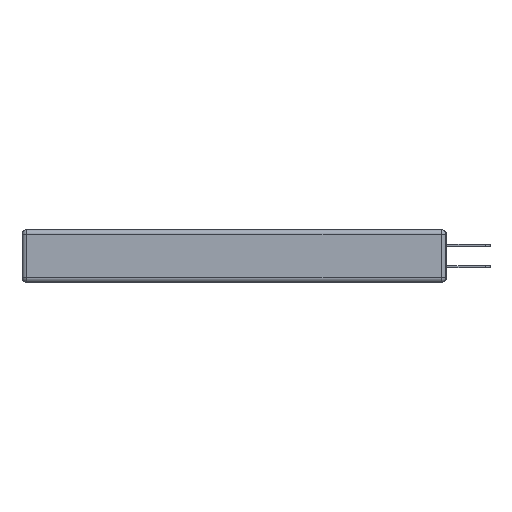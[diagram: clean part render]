
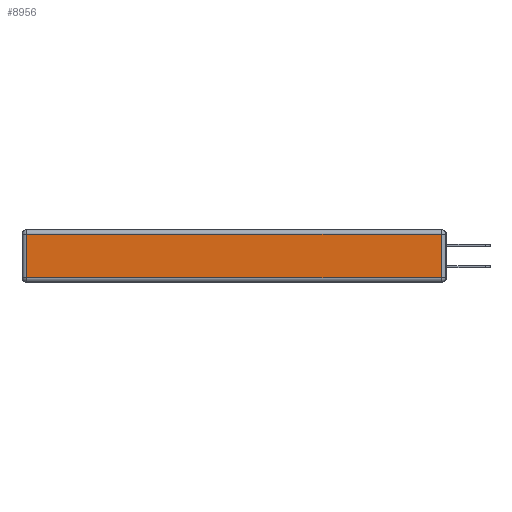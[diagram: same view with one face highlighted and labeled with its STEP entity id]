
A CAD part, left-side view. The second image highlights one B-rep face of the part: STEP entity #8956.
In plain terms, the highlighted planar face has unit normal (-1, 0, 0).
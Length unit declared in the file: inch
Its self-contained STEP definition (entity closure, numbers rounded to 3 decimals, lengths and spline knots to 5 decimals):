
#381 = CARTESIAN_POINT ( 'NONE',  ( 0., 2.72, -0.343 ) ) ;
#869 = DIRECTION ( 'NONE',  ( 0., 0., 1. ) ) ;
#1043 = LINE ( 'NONE', #381, #15610 ) ;
#2469 = DIRECTION ( 'NONE',  ( -1., 0., 0. ) ) ;
#3459 = LINE ( 'NONE', #8683, #8303 ) ;
#4375 = VECTOR ( 'NONE', #24062, 39.37008 ) ;
#4778 = CARTESIAN_POINT ( 'NONE',  ( 0., 2.72, -0.03 ) ) ;
#6944 = AXIS2_PLACEMENT_3D ( 'NONE', #14404, #2469, #7584 ) ;
#7584 = DIRECTION ( 'NONE',  ( 0., 0., 1. ) ) ;
#8303 = VECTOR ( 'NONE', #30071, 39.37008 ) ;
#8683 = CARTESIAN_POINT ( 'NONE',  ( 0., 2.75, -0.03 ) ) ;
#8956 = ADVANCED_FACE ( 'NONE', ( #23258 ), #12391, .T. ) ;
#9294 = EDGE_CURVE ( 'NONE', #21296, #14166, #30298, .T. ) ;
#9839 = CARTESIAN_POINT ( 'NONE',  ( 0., 0., -0.313 ) ) ;
#9922 = DIRECTION ( 'NONE',  ( 0., 0., -1. ) ) ;
#11231 = ORIENTED_EDGE ( 'NONE', *, *, #9294, .T. ) ;
#11254 = VECTOR ( 'NONE', #869, 39.37008 ) ;
#12391 = PLANE ( 'NONE',  #6944 ) ;
#13064 = EDGE_CURVE ( 'NONE', #28808, #21585, #1043, .T. ) ;
#13802 = EDGE_LOOP ( 'NONE', ( #26186, #11231, #14891, #24534 ) ) ;
#14166 = VERTEX_POINT ( 'NONE', #23003 ) ;
#14404 = CARTESIAN_POINT ( 'NONE',  ( 0., 0., -0.343 ) ) ;
#14891 = ORIENTED_EDGE ( 'NONE', *, *, #26861, .T. ) ;
#15610 = VECTOR ( 'NONE', #9922, 39.37008 ) ;
#17410 = CARTESIAN_POINT ( 'NONE',  ( 0., 2.72, -0.313 ) ) ;
#17847 = LINE ( 'NONE', #9839, #4375 ) ;
#19995 = CARTESIAN_POINT ( 'NONE',  ( 0., 0.03, -0.343 ) ) ;
#21296 = VERTEX_POINT ( 'NONE', #25300 ) ;
#21585 = VERTEX_POINT ( 'NONE', #17410 ) ;
#23003 = CARTESIAN_POINT ( 'NONE',  ( 0., 0.03, -0.03 ) ) ;
#23258 = FACE_OUTER_BOUND ( 'NONE', #13802, .T. ) ;
#24062 = DIRECTION ( 'NONE',  ( 0., -1., 0. ) ) ;
#24158 = EDGE_CURVE ( 'NONE', #21585, #21296, #17847, .T. ) ;
#24534 = ORIENTED_EDGE ( 'NONE', *, *, #13064, .T. ) ;
#25300 = CARTESIAN_POINT ( 'NONE',  ( 0., 0.03, -0.313 ) ) ;
#26186 = ORIENTED_EDGE ( 'NONE', *, *, #24158, .T. ) ;
#26861 = EDGE_CURVE ( 'NONE', #14166, #28808, #3459, .T. ) ;
#28808 = VERTEX_POINT ( 'NONE', #4778 ) ;
#30071 = DIRECTION ( 'NONE',  ( 0., 1., 0. ) ) ;
#30298 = LINE ( 'NONE', #19995, #11254 ) ;
